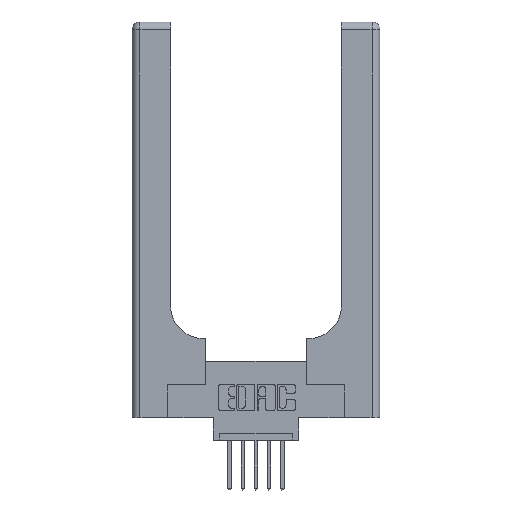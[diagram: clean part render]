
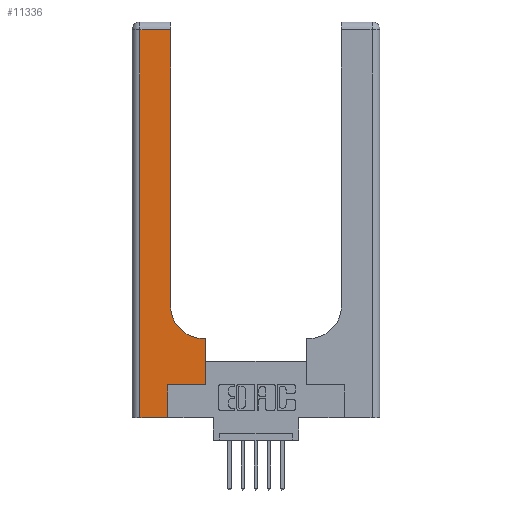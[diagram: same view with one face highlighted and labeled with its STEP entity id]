
A CAD part, top view. The second image highlights one B-rep face of the part: STEP entity #11336.
In plain terms, the highlighted planar face has unit normal (0, 0, 1).
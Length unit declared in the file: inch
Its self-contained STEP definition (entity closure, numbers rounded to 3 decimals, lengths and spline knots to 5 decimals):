
#213 = ORIENTED_EDGE ( 'NONE', *, *, #1803, .T. ) ;
#264 = EDGE_CURVE ( 'NONE', #10613, #10253, #6310, .T. ) ;
#447 = DIRECTION ( 'NONE',  ( -1., 0., 0. ) ) ;
#530 = ORIENTED_EDGE ( 'NONE', *, *, #8611, .T. ) ;
#901 = AXIS2_PLACEMENT_3D ( 'NONE', #12618, #4940, #6172 ) ;
#1187 = CARTESIAN_POINT ( 'NONE',  ( 0.269, 0., 0.37 ) ) ;
#1566 = LINE ( 'NONE', #13416, #9200 ) ;
#1668 = VECTOR ( 'NONE', #6118, 39.37008 ) ;
#1803 = EDGE_CURVE ( 'NONE', #10536, #10613, #8344, .T. ) ;
#1832 = CARTESIAN_POINT ( 'NONE',  ( 0.2915, 0.85, 0.37 ) ) ;
#1858 = VECTOR ( 'NONE', #447, 39.37008 ) ;
#1859 = CARTESIAN_POINT ( 'NONE',  ( 0.2915, 0.6, 0.37 ) ) ;
#2084 = VECTOR ( 'NONE', #13180, 39.37008 ) ;
#2214 = VECTOR ( 'NONE', #7367, 39.37008 ) ;
#2349 = LINE ( 'NONE', #1859, #2865 ) ;
#2600 = LINE ( 'NONE', #1187, #13820 ) ;
#2788 = EDGE_CURVE ( 'NONE', #3967, #5710, #1566, .T. ) ;
#2865 = VECTOR ( 'NONE', #5231, 39.37008 ) ;
#3352 = ORIENTED_EDGE ( 'NONE', *, *, #264, .T. ) ;
#3634 = CARTESIAN_POINT ( 'NONE',  ( 0.5585, 0.25, 0.37 ) ) ;
#3648 = CARTESIAN_POINT ( 'NONE',  ( 0., 2.94, 0.37 ) ) ;
#3650 = EDGE_CURVE ( 'NONE', #11377, #3967, #11745, .T. ) ;
#3904 = ORIENTED_EDGE ( 'NONE', *, *, #3650, .T. ) ;
#3967 = VERTEX_POINT ( 'NONE', #11715 ) ;
#4564 = DIRECTION ( 'NONE',  ( 0., 0., -1. ) ) ;
#4651 = CARTESIAN_POINT ( 'NONE',  ( 0.269, 0.25, 0.37 ) ) ;
#4829 = ORIENTED_EDGE ( 'NONE', *, *, #4885, .T. ) ;
#4885 = EDGE_CURVE ( 'NONE', #10253, #10950, #2349, .T. ) ;
#4940 = DIRECTION ( 'NONE',  ( 0., 0., -1. ) ) ;
#5021 = CARTESIAN_POINT ( 'NONE',  ( 0.2915, 3., 0.37 ) ) ;
#5182 = ORIENTED_EDGE ( 'NONE', *, *, #12181, .T. ) ;
#5231 = DIRECTION ( 'NONE',  ( -1., 0., 0. ) ) ;
#5625 = VECTOR ( 'NONE', #11224, 39.37008 ) ;
#5710 = VERTEX_POINT ( 'NONE', #13425 ) ;
#6040 = FACE_OUTER_BOUND ( 'NONE', #9236, .T. ) ;
#6118 = DIRECTION ( 'NONE',  ( 0., 1., 0. ) ) ;
#6172 = DIRECTION ( 'NONE',  ( -1., 0., 0. ) ) ;
#6310 = LINE ( 'NONE', #3634, #5625 ) ;
#6685 = CARTESIAN_POINT ( 'NONE',  ( 0.5415, 0.85, 0.37 ) ) ;
#6841 = CIRCLE ( 'NONE', #9619, 0.25 ) ;
#7060 = CARTESIAN_POINT ( 'NONE',  ( 0.2915, 2.94, 0.37 ) ) ;
#7367 = DIRECTION ( 'NONE',  ( 0., -1., 0. ) ) ;
#7524 = CARTESIAN_POINT ( 'NONE',  ( 0.5585, 0.6, 0.37 ) ) ;
#7857 = EDGE_CURVE ( 'NONE', #12280, #11377, #9481, .T. ) ;
#8315 = ORIENTED_EDGE ( 'NONE', *, *, #12468, .T. ) ;
#8344 = LINE ( 'NONE', #4651, #2084 ) ;
#8611 = EDGE_CURVE ( 'NONE', #12841, #12280, #13048, .T. ) ;
#8920 = DIRECTION ( 'NONE',  ( 0., 1., 0. ) ) ;
#9200 = VECTOR ( 'NONE', #10045, 39.37008 ) ;
#9236 = EDGE_LOOP ( 'NONE', ( #530, #11456, #3904, #13920, #5182, #213, #3352, #4829, #8315 ) ) ;
#9481 = LINE ( 'NONE', #3648, #1858 ) ;
#9544 = CARTESIAN_POINT ( 'NONE',  ( 0.5585, 0.25, 0.37 ) ) ;
#9619 = AXIS2_PLACEMENT_3D ( 'NONE', #6685, #4564, #10888 ) ;
#10045 = DIRECTION ( 'NONE',  ( 1., 0., 0. ) ) ;
#10253 = VERTEX_POINT ( 'NONE', #7524 ) ;
#10536 = VERTEX_POINT ( 'NONE', #11495 ) ;
#10613 = VERTEX_POINT ( 'NONE', #9544 ) ;
#10625 = CARTESIAN_POINT ( 'NONE',  ( 0.06, 2.94, 0.37 ) ) ;
#10888 = DIRECTION ( 'NONE',  ( 1., 0., 0. ) ) ;
#10950 = VERTEX_POINT ( 'NONE', #13724 ) ;
#11224 = DIRECTION ( 'NONE',  ( 0., 1., 0. ) ) ;
#11336 = ADVANCED_FACE ( 'NONE', ( #6040 ), #11496, .F. ) ;
#11377 = VERTEX_POINT ( 'NONE', #10625 ) ;
#11456 = ORIENTED_EDGE ( 'NONE', *, *, #7857, .T. ) ;
#11495 = CARTESIAN_POINT ( 'NONE',  ( 0.269, 0.25, 0.37 ) ) ;
#11496 = PLANE ( 'NONE',  #901 ) ;
#11715 = CARTESIAN_POINT ( 'NONE',  ( 0.06, 0., 0.37 ) ) ;
#11745 = LINE ( 'NONE', #12853, #2214 ) ;
#12181 = EDGE_CURVE ( 'NONE', #5710, #10536, #2600, .T. ) ;
#12280 = VERTEX_POINT ( 'NONE', #7060 ) ;
#12468 = EDGE_CURVE ( 'NONE', #10950, #12841, #6841, .T. ) ;
#12618 = CARTESIAN_POINT ( 'NONE',  ( 0., 3., 0.37 ) ) ;
#12841 = VERTEX_POINT ( 'NONE', #1832 ) ;
#12853 = CARTESIAN_POINT ( 'NONE',  ( 0.06, 3., 0.37 ) ) ;
#13048 = LINE ( 'NONE', #5021, #1668 ) ;
#13180 = DIRECTION ( 'NONE',  ( 1., 0., 0. ) ) ;
#13416 = CARTESIAN_POINT ( 'NONE',  ( 0., 0., 0.37 ) ) ;
#13425 = CARTESIAN_POINT ( 'NONE',  ( 0.269, 0., 0.37 ) ) ;
#13724 = CARTESIAN_POINT ( 'NONE',  ( 0.5415, 0.6, 0.37 ) ) ;
#13820 = VECTOR ( 'NONE', #8920, 39.37008 ) ;
#13920 = ORIENTED_EDGE ( 'NONE', *, *, #2788, .T. ) ;
